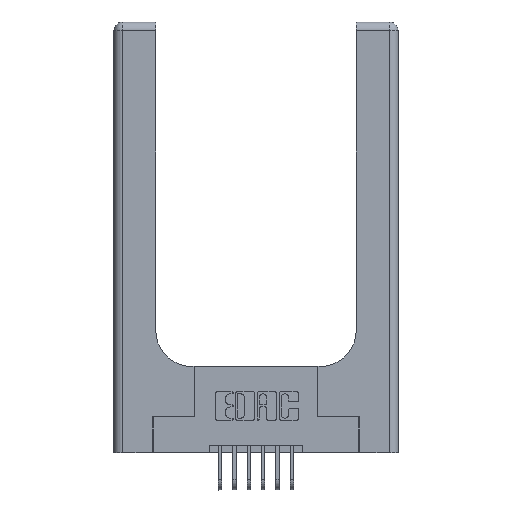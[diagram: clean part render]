
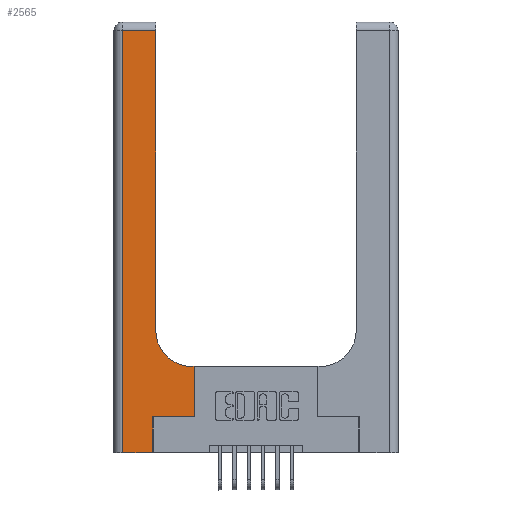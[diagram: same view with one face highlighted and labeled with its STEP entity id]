
A CAD part, top view. The second image highlights one B-rep face of the part: STEP entity #2565.
In plain terms, the highlighted planar face has unit normal (0, 0, 1).
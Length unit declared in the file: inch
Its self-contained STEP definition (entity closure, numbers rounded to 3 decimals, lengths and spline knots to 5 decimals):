
#179 = CIRCLE ( 'NONE', #11237, 0.25 ) ;
#510 = VECTOR ( 'NONE', #14425, 39.37008 ) ;
#547 = LINE ( 'NONE', #13600, #510 ) ;
#564 = VECTOR ( 'NONE', #11766, 39.37008 ) ;
#585 = LINE ( 'NONE', #3714, #564 ) ;
#658 = DIRECTION ( 'NONE',  ( 1., 0., 0. ) ) ;
#702 = FACE_OUTER_BOUND ( 'NONE', #8236, .T. ) ;
#1169 = CARTESIAN_POINT ( 'NONE',  ( 0.2915, 2.94, 0.37 ) ) ;
#1603 = DIRECTION ( 'NONE',  ( 0., 1., 0. ) ) ;
#1851 = EDGE_CURVE ( 'NONE', #9145, #7651, #4952, .T. ) ;
#2382 = ORIENTED_EDGE ( 'NONE', *, *, #10139, .T. ) ;
#2398 = ORIENTED_EDGE ( 'NONE', *, *, #10605, .T. ) ;
#2565 = ADVANCED_FACE ( 'NONE', ( #702 ), #6104, .F. ) ;
#2640 = VERTEX_POINT ( 'NONE', #7493 ) ;
#2651 = LINE ( 'NONE', #2719, #2690 ) ;
#2676 = DIRECTION ( 'NONE',  ( -1., 0., 0. ) ) ;
#2684 = ORIENTED_EDGE ( 'NONE', *, *, #10618, .T. ) ;
#2690 = VECTOR ( 'NONE', #7627, 39.37008 ) ;
#2719 = CARTESIAN_POINT ( 'NONE',  ( 0.2915, 3., 0.37 ) ) ;
#2753 = DIRECTION ( 'NONE',  ( 0., 0., -1. ) ) ;
#2885 = ORIENTED_EDGE ( 'NONE', *, *, #8038, .T. ) ;
#3275 = ORIENTED_EDGE ( 'NONE', *, *, #8808, .T. ) ;
#3323 = ORIENTED_EDGE ( 'NONE', *, *, #8868, .T. ) ;
#3454 = ORIENTED_EDGE ( 'NONE', *, *, #9217, .T. ) ;
#3468 = ORIENTED_EDGE ( 'NONE', *, *, #1851, .T. ) ;
#3525 = CARTESIAN_POINT ( 'NONE',  ( 0., 3., 0.37 ) ) ;
#3582 = CARTESIAN_POINT ( 'NONE',  ( 0., 0., 0.37 ) ) ;
#3714 = CARTESIAN_POINT ( 'NONE',  ( 0., 2.94, 0.37 ) ) ;
#3715 = ORIENTED_EDGE ( 'NONE', *, *, #10691, .T. ) ;
#4683 = DIRECTION ( 'NONE',  ( 0., 1., 0. ) ) ;
#4952 = LINE ( 'NONE', #10037, #5045 ) ;
#5045 = VECTOR ( 'NONE', #2676, 39.37008 ) ;
#5315 = CARTESIAN_POINT ( 'NONE',  ( 0.5415, 0.6, 0.37 ) ) ;
#5571 = CARTESIAN_POINT ( 'NONE',  ( 0.2915, 0.85, 0.37 ) ) ;
#5850 = VECTOR ( 'NONE', #1603, 39.37008 ) ;
#6012 = LINE ( 'NONE', #10244, #5850 ) ;
#6104 = PLANE ( 'NONE',  #7507 ) ;
#6157 = DIRECTION ( 'NONE',  ( 1., 0., 0. ) ) ;
#7116 = LINE ( 'NONE', #8538, #7164 ) ;
#7164 = VECTOR ( 'NONE', #658, 39.37008 ) ;
#7213 = CARTESIAN_POINT ( 'NONE',  ( 0.269, 0., 0.37 ) ) ;
#7343 = DIRECTION ( 'NONE',  ( -1., 0., 0. ) ) ;
#7443 = LINE ( 'NONE', #7213, #7502 ) ;
#7493 = CARTESIAN_POINT ( 'NONE',  ( 0.5585, 0.25, 0.37 ) ) ;
#7502 = VECTOR ( 'NONE', #4683, 39.37008 ) ;
#7507 = AXIS2_PLACEMENT_3D ( 'NONE', #3525, #13450, #7343 ) ;
#7627 = DIRECTION ( 'NONE',  ( 0., 1., 0. ) ) ;
#7651 = VERTEX_POINT ( 'NONE', #5315 ) ;
#7745 = VERTEX_POINT ( 'NONE', #13898 ) ;
#7813 = CARTESIAN_POINT ( 'NONE',  ( 0.06, 2.94, 0.37 ) ) ;
#8038 = EDGE_CURVE ( 'NONE', #13907, #7745, #11610, .T. ) ;
#8236 = EDGE_LOOP ( 'NONE', ( #2382, #2398, #2684, #2885, #3275, #3323, #3454, #3468, #3715 ) ) ;
#8538 = CARTESIAN_POINT ( 'NONE',  ( 0.269, 0.25, 0.37 ) ) ;
#8808 = EDGE_CURVE ( 'NONE', #7745, #14170, #7443, .T. ) ;
#8868 = EDGE_CURVE ( 'NONE', #14170, #2640, #7116, .T. ) ;
#9056 = VERTEX_POINT ( 'NONE', #7813 ) ;
#9145 = VERTEX_POINT ( 'NONE', #13864 ) ;
#9217 = EDGE_CURVE ( 'NONE', #2640, #9145, #6012, .T. ) ;
#9560 = CARTESIAN_POINT ( 'NONE',  ( 0.06, 0., 0.37 ) ) ;
#10037 = CARTESIAN_POINT ( 'NONE',  ( 0.2915, 0.6, 0.37 ) ) ;
#10094 = CARTESIAN_POINT ( 'NONE',  ( 0.5415, 0.85, 0.37 ) ) ;
#10139 = EDGE_CURVE ( 'NONE', #11798, #11390, #2651, .T. ) ;
#10244 = CARTESIAN_POINT ( 'NONE',  ( 0.5585, 0.25, 0.37 ) ) ;
#10438 = VECTOR ( 'NONE', #6157, 39.37008 ) ;
#10605 = EDGE_CURVE ( 'NONE', #11390, #9056, #585, .T. ) ;
#10618 = EDGE_CURVE ( 'NONE', #9056, #13907, #547, .T. ) ;
#10691 = EDGE_CURVE ( 'NONE', #7651, #11798, #179, .T. ) ;
#11048 = DIRECTION ( 'NONE',  ( 1., 0., 0. ) ) ;
#11237 = AXIS2_PLACEMENT_3D ( 'NONE', #10094, #2753, #11048 ) ;
#11390 = VERTEX_POINT ( 'NONE', #1169 ) ;
#11610 = LINE ( 'NONE', #3582, #10438 ) ;
#11727 = CARTESIAN_POINT ( 'NONE',  ( 0.269, 0.25, 0.37 ) ) ;
#11766 = DIRECTION ( 'NONE',  ( -1., 0., 0. ) ) ;
#11798 = VERTEX_POINT ( 'NONE', #5571 ) ;
#13450 = DIRECTION ( 'NONE',  ( 0., 0., -1. ) ) ;
#13600 = CARTESIAN_POINT ( 'NONE',  ( 0.06, 3., 0.37 ) ) ;
#13864 = CARTESIAN_POINT ( 'NONE',  ( 0.5585, 0.6, 0.37 ) ) ;
#13898 = CARTESIAN_POINT ( 'NONE',  ( 0.269, 0., 0.37 ) ) ;
#13907 = VERTEX_POINT ( 'NONE', #9560 ) ;
#14170 = VERTEX_POINT ( 'NONE', #11727 ) ;
#14425 = DIRECTION ( 'NONE',  ( 0., -1., 0. ) ) ;
